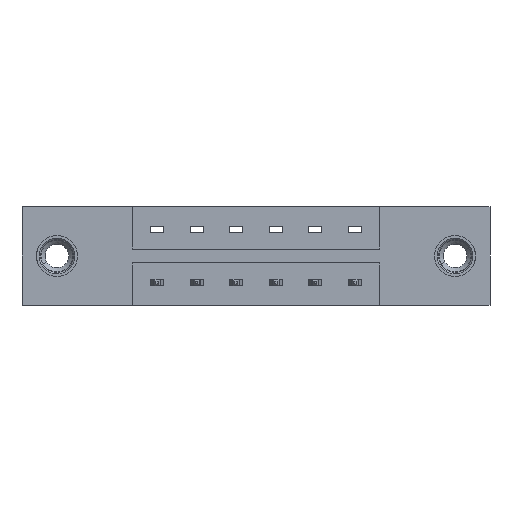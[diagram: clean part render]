
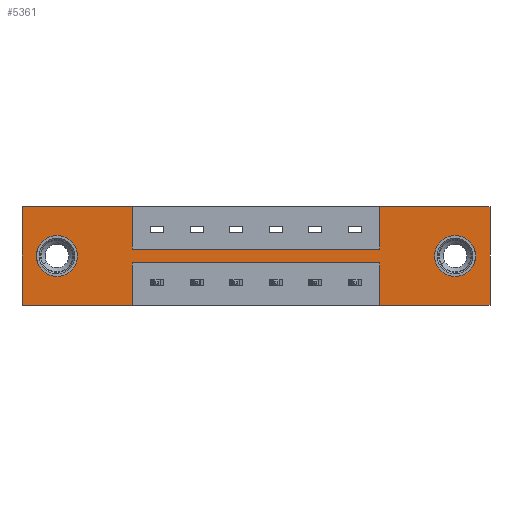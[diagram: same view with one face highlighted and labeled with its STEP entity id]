
A CAD part, front view. The second image highlights one B-rep face of the part: STEP entity #5361.
In plain terms, the highlighted planar face has unit normal (0, -1, 0).
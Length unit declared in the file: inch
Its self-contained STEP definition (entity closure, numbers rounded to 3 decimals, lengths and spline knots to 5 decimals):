
#6 = EDGE_CURVE ( 'NONE', #7616, #4328, #9257, .T. ) ;
#9 = CARTESIAN_POINT ( 'NONE',  ( 0.4175, 0., 0. ) ) ;
#24 = FACE_OUTER_BOUND ( 'NONE', #7587, .T. ) ;
#120 = ORIENTED_EDGE ( 'NONE', *, *, #5979, .F. ) ;
#211 = CARTESIAN_POINT ( 'NONE',  ( 1.3575, 0., -0.214 ) ) ;
#242 = LINE ( 'NONE', #5308, #1256 ) ;
#365 = CARTESIAN_POINT ( 'NONE',  ( 1.6425, 0., -0.2655 ) ) ;
#390 = ORIENTED_EDGE ( 'NONE', *, *, #6316, .F. ) ;
#411 = DIRECTION ( 'NONE',  ( 0., 0., 1. ) ) ;
#456 = CARTESIAN_POINT ( 'NONE',  ( 0.1325, 0., -0.1875 ) ) ;
#498 = FACE_BOUND ( 'NONE', #9178, .T. ) ;
#791 = CARTESIAN_POINT ( 'NONE',  ( 0.4175, 0., -0.214 ) ) ;
#892 = DIRECTION ( 'NONE',  ( 0., 0., -1. ) ) ;
#965 = EDGE_CURVE ( 'NONE', #9172, #5314, #7655, .T. ) ;
#982 = DIRECTION ( 'NONE',  ( 0., 0., -1. ) ) ;
#1034 = CARTESIAN_POINT ( 'NONE',  ( 0.4175, 0., -0.161 ) ) ;
#1067 = DIRECTION ( 'NONE',  ( 0., 0., -1. ) ) ;
#1083 = DIRECTION ( 'NONE',  ( 1., 0., 0. ) ) ;
#1097 = CIRCLE ( 'NONE', #9357, 0.078 ) ;
#1106 = ORIENTED_EDGE ( 'NONE', *, *, #9453, .F. ) ;
#1255 = ORIENTED_EDGE ( 'NONE', *, *, #965, .F. ) ;
#1256 = VECTOR ( 'NONE', #892, 39.37008 ) ;
#1426 = CARTESIAN_POINT ( 'NONE',  ( 1.6425, 0., -0.1875 ) ) ;
#1456 = DIRECTION ( 'NONE',  ( 0., 0., -1. ) ) ;
#1463 = LINE ( 'NONE', #2580, #7146 ) ;
#1515 = CARTESIAN_POINT ( 'NONE',  ( 1.6425, 0., -0.1095 ) ) ;
#1540 = ORIENTED_EDGE ( 'NONE', *, *, #4158, .T. ) ;
#1691 = LINE ( 'NONE', #3917, #6332 ) ;
#1709 = CARTESIAN_POINT ( 'NONE',  ( 1.775, 0., 0. ) ) ;
#1790 = VECTOR ( 'NONE', #4322, 39.37008 ) ;
#1814 = DIRECTION ( 'NONE',  ( 0., -1., 0. ) ) ;
#1965 = EDGE_LOOP ( 'NONE', ( #7043, #1540 ) ) ;
#1994 = VERTEX_POINT ( 'NONE', #6394 ) ;
#2161 = CARTESIAN_POINT ( 'NONE',  ( 0., 0., 0. ) ) ;
#2259 = VERTEX_POINT ( 'NONE', #7512 ) ;
#2302 = LINE ( 'NONE', #6621, #3916 ) ;
#2357 = AXIS2_PLACEMENT_3D ( 'NONE', #1426, #2921, #1456 ) ;
#2391 = CARTESIAN_POINT ( 'NONE',  ( 1.6425, 0., -0.1875 ) ) ;
#2399 = VERTEX_POINT ( 'NONE', #3154 ) ;
#2580 = CARTESIAN_POINT ( 'NONE',  ( 1.3575, 0., -0.161 ) ) ;
#2710 = DIRECTION ( 'NONE',  ( 0., 0., 1. ) ) ;
#2742 = EDGE_CURVE ( 'NONE', #4328, #7616, #9422, .T. ) ;
#2833 = VERTEX_POINT ( 'NONE', #211 ) ;
#2908 = VERTEX_POINT ( 'NONE', #6983 ) ;
#2921 = DIRECTION ( 'NONE',  ( 0., 1., 0. ) ) ;
#3154 = CARTESIAN_POINT ( 'NONE',  ( 0.4175, 0., -0.214 ) ) ;
#3184 = EDGE_CURVE ( 'NONE', #8688, #9172, #4436, .T. ) ;
#3248 = CARTESIAN_POINT ( 'NONE',  ( 0.4175, 0., -0.161 ) ) ;
#3377 = VERTEX_POINT ( 'NONE', #7394 ) ;
#3417 = DIRECTION ( 'NONE',  ( 0., 1., 0. ) ) ;
#3506 = LINE ( 'NONE', #9552, #4549 ) ;
#3579 = DIRECTION ( 'NONE',  ( -1., 0., 0. ) ) ;
#3702 = CARTESIAN_POINT ( 'NONE',  ( 1.3575, 0., -0.214 ) ) ;
#3797 = AXIS2_PLACEMENT_3D ( 'NONE', #9242, #1814, #1067 ) ;
#3860 = EDGE_CURVE ( 'NONE', #5836, #2833, #5381, .T. ) ;
#3916 = VECTOR ( 'NONE', #8147, 39.37008 ) ;
#3917 = CARTESIAN_POINT ( 'NONE',  ( 0.4175, 0., -0.161 ) ) ;
#3947 = DIRECTION ( 'NONE',  ( 1., 0., 0. ) ) ;
#3957 = ORIENTED_EDGE ( 'NONE', *, *, #8038, .F. ) ;
#4102 = ORIENTED_EDGE ( 'NONE', *, *, #8747, .F. ) ;
#4158 = EDGE_CURVE ( 'NONE', #8832, #2908, #1097, .T. ) ;
#4269 = EDGE_CURVE ( 'NONE', #2833, #2399, #8937, .T. ) ;
#4317 = VECTOR ( 'NONE', #982, 39.37008 ) ;
#4322 = DIRECTION ( 'NONE',  ( 1., 0., 0. ) ) ;
#4328 = VERTEX_POINT ( 'NONE', #1515 ) ;
#4436 = LINE ( 'NONE', #2161, #1790 ) ;
#4549 = VECTOR ( 'NONE', #3579, 39.37008 ) ;
#4614 = EDGE_CURVE ( 'NONE', #3377, #8253, #8273, .T. ) ;
#4804 = CARTESIAN_POINT ( 'NONE',  ( 0., 0., 0. ) ) ;
#4941 = VECTOR ( 'NONE', #8445, 39.37008 ) ;
#5130 = VECTOR ( 'NONE', #7417, 39.37008 ) ;
#5145 = AXIS2_PLACEMENT_3D ( 'NONE', #2391, #8335, #9051 ) ;
#5308 = CARTESIAN_POINT ( 'NONE',  ( 0.4175, 0., -0.214 ) ) ;
#5314 = VERTEX_POINT ( 'NONE', #1034 ) ;
#5361 = ADVANCED_FACE ( 'NONE', ( #498, #6147, #24 ), #5488, .T. ) ;
#5381 = LINE ( 'NONE', #3702, #7595 ) ;
#5440 = CARTESIAN_POINT ( 'NONE',  ( 0., 0., 0. ) ) ;
#5488 = PLANE ( 'NONE',  #3797 ) ;
#5607 = VERTEX_POINT ( 'NONE', #8719 ) ;
#5836 = VERTEX_POINT ( 'NONE', #6867 ) ;
#5979 = EDGE_CURVE ( 'NONE', #1994, #3377, #8890, .T. ) ;
#6068 = ORIENTED_EDGE ( 'NONE', *, *, #3184, .F. ) ;
#6147 = FACE_BOUND ( 'NONE', #1965, .T. ) ;
#6177 = CARTESIAN_POINT ( 'NONE',  ( 0., 0., -0.375 ) ) ;
#6316 = EDGE_CURVE ( 'NONE', #2259, #8688, #2302, .T. ) ;
#6332 = VECTOR ( 'NONE', #3947, 39.37008 ) ;
#6359 = VECTOR ( 'NONE', #7620, 39.37008 ) ;
#6367 = CARTESIAN_POINT ( 'NONE',  ( 0.1325, 0., -0.2655 ) ) ;
#6394 = CARTESIAN_POINT ( 'NONE',  ( 1.3575, 0., 0. ) ) ;
#6621 = CARTESIAN_POINT ( 'NONE',  ( 0., 0., 0. ) ) ;
#6705 = VECTOR ( 'NONE', #1083, 39.37008 ) ;
#6800 = EDGE_CURVE ( 'NONE', #2399, #5607, #242, .T. ) ;
#6867 = CARTESIAN_POINT ( 'NONE',  ( 1.3575, 0., -0.375 ) ) ;
#6911 = EDGE_CURVE ( 'NONE', #8253, #5836, #6933, .T. ) ;
#6933 = LINE ( 'NONE', #6177, #4941 ) ;
#6983 = CARTESIAN_POINT ( 'NONE',  ( 0.1325, 0., -0.1095 ) ) ;
#7043 = ORIENTED_EDGE ( 'NONE', *, *, #8278, .T. ) ;
#7144 = CIRCLE ( 'NONE', #7302, 0.078 ) ;
#7146 = VECTOR ( 'NONE', #411, 39.37008 ) ;
#7302 = AXIS2_PLACEMENT_3D ( 'NONE', #456, #3417, #2710 ) ;
#7394 = CARTESIAN_POINT ( 'NONE',  ( 1.775, 0., 0. ) ) ;
#7417 = DIRECTION ( 'NONE',  ( -1., 0., 0. ) ) ;
#7512 = CARTESIAN_POINT ( 'NONE',  ( 0., 0., -0.375 ) ) ;
#7587 = EDGE_LOOP ( 'NONE', ( #8539, #8689, #8048, #120, #4102, #3957, #1255, #6068, #390, #1106, #7699, #7666 ) ) ;
#7595 = VECTOR ( 'NONE', #8879, 39.37008 ) ;
#7616 = VERTEX_POINT ( 'NONE', #365 ) ;
#7620 = DIRECTION ( 'NONE',  ( 0., 0., -1. ) ) ;
#7655 = LINE ( 'NONE', #3248, #6359 ) ;
#7666 = ORIENTED_EDGE ( 'NONE', *, *, #4269, .F. ) ;
#7699 = ORIENTED_EDGE ( 'NONE', *, *, #6800, .F. ) ;
#7813 = ORIENTED_EDGE ( 'NONE', *, *, #6, .T. ) ;
#8038 = EDGE_CURVE ( 'NONE', #5314, #9423, #1691, .T. ) ;
#8048 = ORIENTED_EDGE ( 'NONE', *, *, #4614, .F. ) ;
#8147 = DIRECTION ( 'NONE',  ( 0., 0., 1. ) ) ;
#8253 = VERTEX_POINT ( 'NONE', #8667 ) ;
#8273 = LINE ( 'NONE', #1709, #4317 ) ;
#8278 = EDGE_CURVE ( 'NONE', #2908, #8832, #7144, .T. ) ;
#8335 = DIRECTION ( 'NONE',  ( 0., 1., 0. ) ) ;
#8445 = DIRECTION ( 'NONE',  ( -1., 0., 0. ) ) ;
#8539 = ORIENTED_EDGE ( 'NONE', *, *, #3860, .F. ) ;
#8635 = CARTESIAN_POINT ( 'NONE',  ( 0.1325, 0., -0.1875 ) ) ;
#8667 = CARTESIAN_POINT ( 'NONE',  ( 1.775, 0., -0.375 ) ) ;
#8685 = DIRECTION ( 'NONE',  ( 0., 0., 1. ) ) ;
#8688 = VERTEX_POINT ( 'NONE', #5440 ) ;
#8689 = ORIENTED_EDGE ( 'NONE', *, *, #6911, .F. ) ;
#8719 = CARTESIAN_POINT ( 'NONE',  ( 0.4175, 0., -0.375 ) ) ;
#8724 = ORIENTED_EDGE ( 'NONE', *, *, #2742, .T. ) ;
#8747 = EDGE_CURVE ( 'NONE', #9423, #1994, #1463, .T. ) ;
#8832 = VERTEX_POINT ( 'NONE', #6367 ) ;
#8879 = DIRECTION ( 'NONE',  ( 0., 0., 1. ) ) ;
#8890 = LINE ( 'NONE', #4804, #6705 ) ;
#8937 = LINE ( 'NONE', #791, #5130 ) ;
#9051 = DIRECTION ( 'NONE',  ( 0., 0., -1. ) ) ;
#9172 = VERTEX_POINT ( 'NONE', #9 ) ;
#9178 = EDGE_LOOP ( 'NONE', ( #8724, #7813 ) ) ;
#9242 = CARTESIAN_POINT ( 'NONE',  ( 0., 0., -0.375 ) ) ;
#9257 = CIRCLE ( 'NONE', #5145, 0.078 ) ;
#9357 = AXIS2_PLACEMENT_3D ( 'NONE', #8635, #9358, #8685 ) ;
#9358 = DIRECTION ( 'NONE',  ( 0., 1., 0. ) ) ;
#9422 = CIRCLE ( 'NONE', #2357, 0.078 ) ;
#9423 = VERTEX_POINT ( 'NONE', #9426 ) ;
#9426 = CARTESIAN_POINT ( 'NONE',  ( 1.3575, 0., -0.161 ) ) ;
#9453 = EDGE_CURVE ( 'NONE', #5607, #2259, #3506, .T. ) ;
#9552 = CARTESIAN_POINT ( 'NONE',  ( 0., 0., -0.375 ) ) ;
